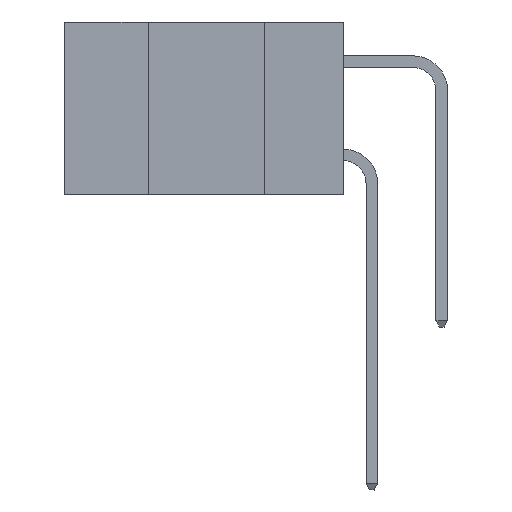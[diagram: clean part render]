
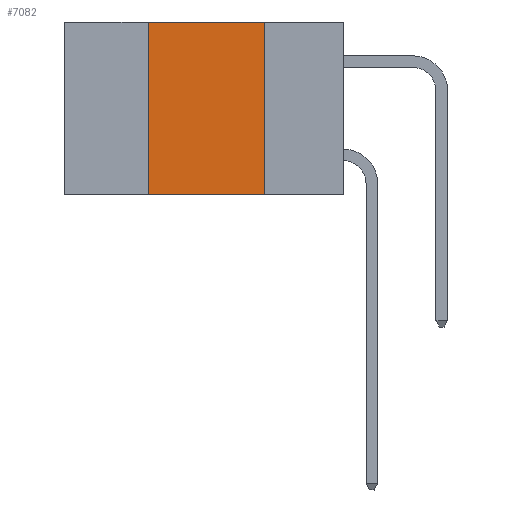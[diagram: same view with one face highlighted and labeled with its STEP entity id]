
A CAD part, left-side view. The second image highlights one B-rep face of the part: STEP entity #7082.
In plain terms, the highlighted planar face has unit normal (-1, 0, 0).
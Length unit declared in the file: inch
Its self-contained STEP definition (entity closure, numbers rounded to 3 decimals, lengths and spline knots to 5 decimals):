
#1313 = LINE ( 'NONE', #5818, #19488 ) ;
#1878 = ORIENTED_EDGE ( 'NONE', *, *, #9905, .F. ) ;
#2709 = CARTESIAN_POINT ( 'NONE',  ( 0., 0.17, 0. ) ) ;
#3889 = EDGE_CURVE ( 'NONE', #21096, #12744, #15368, .T. ) ;
#4049 = DIRECTION ( 'NONE',  ( 0., 0., -1. ) ) ;
#4065 = CARTESIAN_POINT ( 'NONE',  ( 0., 0.6, 0. ) ) ;
#4137 = LINE ( 'NONE', #15217, #21759 ) ;
#5818 = CARTESIAN_POINT ( 'NONE',  ( 0., 0.17, 0. ) ) ;
#5831 = DIRECTION ( 'NONE',  ( 0., 0., -1. ) ) ;
#6403 = LINE ( 'NONE', #7229, #15215 ) ;
#7082 = ADVANCED_FACE ( 'NONE', ( #16891 ), #21606, .F. ) ;
#7229 = CARTESIAN_POINT ( 'NONE',  ( 0., 0.42, 0. ) ) ;
#7630 = EDGE_CURVE ( 'NONE', #12312, #21096, #6403, .T. ) ;
#7746 = CARTESIAN_POINT ( 'NONE',  ( 0., 0.42, 0. ) ) ;
#8413 = DIRECTION ( 'NONE',  ( 0., -1., 0. ) ) ;
#9905 = EDGE_CURVE ( 'NONE', #12744, #17280, #1313, .T. ) ;
#11237 = ORIENTED_EDGE ( 'NONE', *, *, #3889, .F. ) ;
#11797 = ORIENTED_EDGE ( 'NONE', *, *, #7630, .F. ) ;
#12223 = EDGE_LOOP ( 'NONE', ( #1878, #11237, #11797, #17032 ) ) ;
#12312 = VERTEX_POINT ( 'NONE', #16198 ) ;
#12744 = VERTEX_POINT ( 'NONE', #2709 ) ;
#13500 = EDGE_CURVE ( 'NONE', #12312, #17280, #4137, .T. ) ;
#15215 = VECTOR ( 'NONE', #21294, 39.37008 ) ;
#15217 = CARTESIAN_POINT ( 'NONE',  ( 0., 0.6, -0.37 ) ) ;
#15368 = LINE ( 'NONE', #20716, #20051 ) ;
#16198 = CARTESIAN_POINT ( 'NONE',  ( 0., 0.42, -0.37 ) ) ;
#16377 = DIRECTION ( 'NONE',  ( 1., 0., 0. ) ) ;
#16891 = FACE_OUTER_BOUND ( 'NONE', #12223, .T. ) ;
#16975 = CARTESIAN_POINT ( 'NONE',  ( 0., 0.17, -0.37 ) ) ;
#16999 = DIRECTION ( 'NONE',  ( 0., -1., 0. ) ) ;
#17032 = ORIENTED_EDGE ( 'NONE', *, *, #13500, .T. ) ;
#17280 = VERTEX_POINT ( 'NONE', #16975 ) ;
#19488 = VECTOR ( 'NONE', #4049, 39.37008 ) ;
#19850 = AXIS2_PLACEMENT_3D ( 'NONE', #4065, #16377, #5831 ) ;
#20051 = VECTOR ( 'NONE', #8413, 39.37008 ) ;
#20716 = CARTESIAN_POINT ( 'NONE',  ( 0., 0.6, 0. ) ) ;
#21096 = VERTEX_POINT ( 'NONE', #7746 ) ;
#21294 = DIRECTION ( 'NONE',  ( 0., 0., 1. ) ) ;
#21606 = PLANE ( 'NONE',  #19850 ) ;
#21759 = VECTOR ( 'NONE', #16999, 39.37008 ) ;
